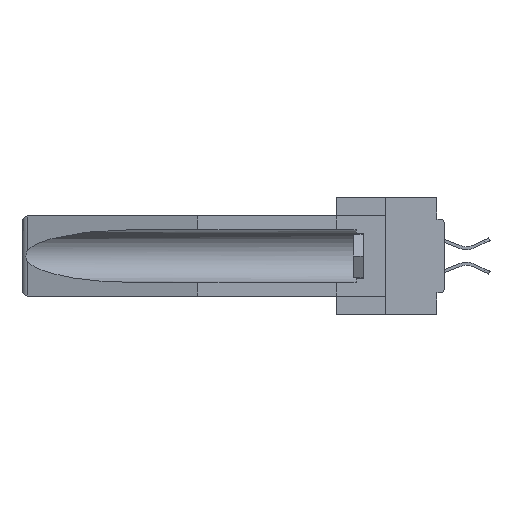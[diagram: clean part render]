
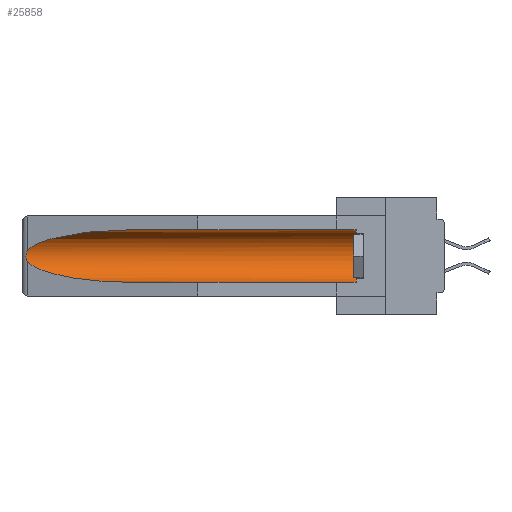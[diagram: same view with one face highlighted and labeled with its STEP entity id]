
A CAD part, left-side view. The second image highlights one B-rep face of the part: STEP entity #25858.
In plain terms, the highlighted cylindrical face has radius 2.857 mm (diameter 5.715 mm), a partial arc.
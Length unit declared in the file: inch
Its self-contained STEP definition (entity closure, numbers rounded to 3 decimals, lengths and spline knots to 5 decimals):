
#373 = EDGE_CURVE ( 'NONE', #22749, #5772, #42729, .T. ) ;
#486 =( BOUNDED_CURVE ( )  B_SPLINE_CURVE ( 3, ( #1019, #11566, #22351, #4700 ),
 .UNSPECIFIED., .F., .T. ) 
 B_SPLINE_CURVE_WITH_KNOTS ( ( 4, 4 ),
 ( 4.71239, 6.08839 ),
 .UNSPECIFIED. ) 
 CURVE ( )  GEOMETRIC_REPRESENTATION_ITEM ( )  RATIONAL_B_SPLINE_CURVE ( ( 1., 0.848, 0.848, 1. ) ) 
 REPRESENTATION_ITEM ( '' )  );
#1019 = CARTESIAN_POINT ( 'NONE',  ( 0.155, 1.07973, -0.059 ) ) ;
#2647 = CARTESIAN_POINT ( 'NONE',  ( 0.155, -0.30754, -0.284 ) ) ;
#3547 = ORIENTED_EDGE ( 'NONE', *, *, #24380, .T. ) ;
#4700 = CARTESIAN_POINT ( 'NONE',  ( 0.26537, 1.52718, -0.14972 ) ) ;
#4844 = CARTESIAN_POINT ( 'NONE',  ( 0.155, 0.126, -0.284 ) ) ;
#4983 = ORIENTED_EDGE ( 'NONE', *, *, #42241, .F. ) ;
#5086 = VERTEX_POINT ( 'NONE', #11338 ) ;
#5247 = CARTESIAN_POINT ( 'NONE',  ( 0.2673, 1.5327, -0.16383 ) ) ;
#5772 = VERTEX_POINT ( 'NONE', #16551 ) ;
#6023 = VERTEX_POINT ( 'NONE', #33227 ) ;
#7789 = ORIENTED_EDGE ( 'NONE', *, *, #373, .T. ) ;
#8074 = VERTEX_POINT ( 'NONE', #24790 ) ;
#8927 = CARTESIAN_POINT ( 'NONE',  ( 0.26597, 1.52961, -0.15275 ) ) ;
#9375 = CARTESIAN_POINT ( 'NONE',  ( 0.26537, 1.52718, -0.19328 ) ) ;
#10784 = DIRECTION ( 'NONE',  ( 0., 0., 1. ) ) ;
#11338 = CARTESIAN_POINT ( 'NONE',  ( 0.155, 1.07973, -0.284 ) ) ;
#11432 = ORIENTED_EDGE ( 'NONE', *, *, #42269, .T. ) ;
#11566 = CARTESIAN_POINT ( 'NONE',  ( 0.21114, 1.30732, -0.059 ) ) ;
#12592 = CARTESIAN_POINT ( 'NONE',  ( 0.26655, 1.53094, -0.18657 ) ) ;
#12751 = CARTESIAN_POINT ( 'NONE',  ( 0.26537, 1.52718, -0.14972 ) ) ;
#12906 = CARTESIAN_POINT ( 'NONE',  ( 0.2675, 1.53308, -0.17534 ) ) ;
#12924 = EDGE_CURVE ( 'NONE', #27542, #5086, #34351, .T. ) ;
#13191 = CARTESIAN_POINT ( 'NONE',  ( 0.21114, 1.30732, -0.284 ) ) ;
#15865 = AXIS2_PLACEMENT_3D ( 'NONE', #29058, #43819, #10784 ) ;
#16551 = CARTESIAN_POINT ( 'NONE',  ( 0.155, 0.126, -0.059 ) ) ;
#16660 = CARTESIAN_POINT ( 'NONE',  ( 0.155, 1.07973, -0.284 ) ) ;
#17099 = VECTOR ( 'NONE', #36002, 39.37008 ) ;
#17231 = DIRECTION ( 'NONE',  ( 0., 0., 1. ) ) ;
#20029 = VECTOR ( 'NONE', #31901, 39.37008 ) ;
#21177 = LINE ( 'NONE', #2647, #20029 ) ;
#22351 = CARTESIAN_POINT ( 'NONE',  ( 0.25451, 1.48313, -0.09465 ) ) ;
#22511 = ORIENTED_EDGE ( 'NONE', *, *, #12924, .T. ) ;
#22749 = VERTEX_POINT ( 'NONE', #4844 ) ;
#24380 = EDGE_CURVE ( 'NONE', #5772, #6023, #36463, .T. ) ;
#24790 = CARTESIAN_POINT ( 'NONE',  ( 0.26537, 1.52718, -0.14972 ) ) ;
#24863 = DIRECTION ( 'NONE',  ( 0., -1., 0. ) ) ;
#25858 = ADVANCED_FACE ( 'NONE', ( #43210 ), #44947, .F. ) ;
#26887 = CARTESIAN_POINT ( 'NONE',  ( 0.26654, 1.53092, -0.15636 ) ) ;
#27542 = VERTEX_POINT ( 'NONE', #29780 ) ;
#27633 = CARTESIAN_POINT ( 'NONE',  ( 0.25451, 1.48313, -0.24835 ) ) ;
#29058 = CARTESIAN_POINT ( 'NONE',  ( 0.155, -0.30754, -0.1715 ) ) ;
#29780 = CARTESIAN_POINT ( 'NONE',  ( 0.26537, 1.52718, -0.19328 ) ) ;
#31901 = DIRECTION ( 'NONE',  ( 0., 1., 0. ) ) ;
#33227 = CARTESIAN_POINT ( 'NONE',  ( 0.155, 1.07973, -0.059 ) ) ;
#34216 = CARTESIAN_POINT ( 'NONE',  ( 0.2675, 1.53308, -0.16763 ) ) ;
#34351 =( BOUNDED_CURVE ( )  B_SPLINE_CURVE ( 3, ( #9375, #27633, #13191, #16660 ),
 .UNSPECIFIED., .F., .F. ) 
 B_SPLINE_CURVE_WITH_KNOTS ( ( 4, 4 ),
 ( 0.1948, 1.5708 ),
 .UNSPECIFIED. ) 
 CURVE ( )  GEOMETRIC_REPRESENTATION_ITEM ( )  RATIONAL_B_SPLINE_CURVE ( ( 1., 0.848, 0.848, 1. ) ) 
 REPRESENTATION_ITEM ( '' )  );
#34369 = CARTESIAN_POINT ( 'NONE',  ( 0.2673, 1.53269, -0.17917 ) ) ;
#35100 = EDGE_LOOP ( 'NONE', ( #11432, #46473, #22511, #4983, #7789, #3547 ) ) ;
#35196 = B_SPLINE_CURVE_WITH_KNOTS ( 'NONE', 3,
 ( #12751, #8927, #26887, #5247, #34216, #12906, #34369, #12592, #45467, #45643 ),
 .UNSPECIFIED., .F., .F.,
 ( 4, 2, 2, 2, 4 ),
 ( 0., 0.00029, 0.00058, 0.00087, 0.00117 ),
 .UNSPECIFIED. ) ;
#36002 = DIRECTION ( 'NONE',  ( 0., 1., 0. ) ) ;
#36463 = LINE ( 'NONE', #43459, #17099 ) ;
#36932 = EDGE_CURVE ( 'NONE', #8074, #27542, #35196, .T. ) ;
#41596 = AXIS2_PLACEMENT_3D ( 'NONE', #46661, #24863, #17231 ) ;
#42241 = EDGE_CURVE ( 'NONE', #22749, #5086, #21177, .T. ) ;
#42269 = EDGE_CURVE ( 'NONE', #6023, #8074, #486, .T. ) ;
#42729 = CIRCLE ( 'NONE', #41596, 0.1125 ) ;
#43210 = FACE_OUTER_BOUND ( 'NONE', #35100, .T. ) ;
#43459 = CARTESIAN_POINT ( 'NONE',  ( 0.155, -0.30754, -0.059 ) ) ;
#43819 = DIRECTION ( 'NONE',  ( 0., 1., 0. ) ) ;
#44947 = CYLINDRICAL_SURFACE ( 'NONE', #15865, 0.1125 ) ;
#45467 = CARTESIAN_POINT ( 'NONE',  ( 0.26597, 1.5296, -0.19026 ) ) ;
#45643 = CARTESIAN_POINT ( 'NONE',  ( 0.26537, 1.52718, -0.19328 ) ) ;
#46473 = ORIENTED_EDGE ( 'NONE', *, *, #36932, .T. ) ;
#46661 = CARTESIAN_POINT ( 'NONE',  ( 0.155, 0.126, -0.1715 ) ) ;
